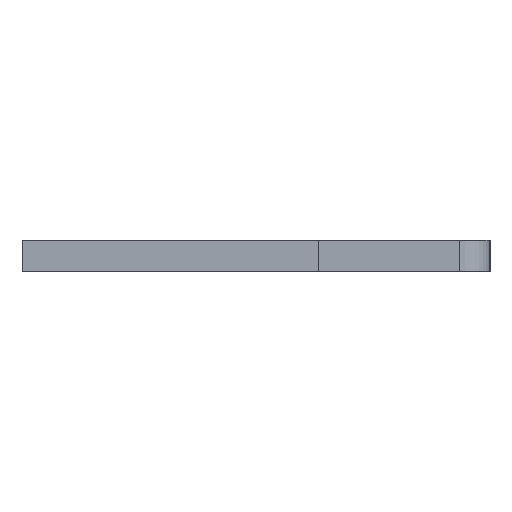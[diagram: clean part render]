
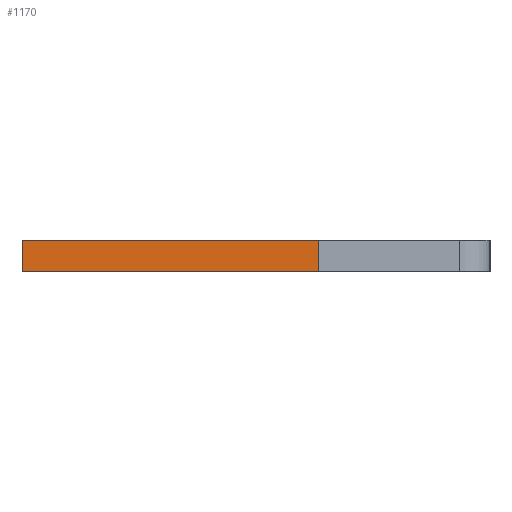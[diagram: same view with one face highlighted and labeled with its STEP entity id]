
A CAD part, left-side view. The second image highlights one B-rep face of the part: STEP entity #1170.
In plain terms, the highlighted face is planar.
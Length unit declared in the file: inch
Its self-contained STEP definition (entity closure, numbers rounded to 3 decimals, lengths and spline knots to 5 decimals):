
#12 = PLANE ( 'NONE',  #381 ) ;
#14 = EDGE_CURVE ( 'NONE', #1095, #1069, #570, .T. ) ;
#95 = DIRECTION ( 'NONE',  ( 0., 1., 0. ) ) ;
#118 = DIRECTION ( 'NONE',  ( 0., 1., 0. ) ) ;
#135 = VECTOR ( 'NONE', #1110, 39.37008 ) ;
#197 = DIRECTION ( 'NONE',  ( 1., 0., 0. ) ) ;
#214 = CARTESIAN_POINT ( 'NONE',  ( 0.01, -0.04, -0.04 ) ) ;
#228 = VECTOR ( 'NONE', #118, 39.37008 ) ;
#239 = DIRECTION ( 'NONE',  ( -1., 0., 0. ) ) ;
#285 = CARTESIAN_POINT ( 'NONE',  ( 0.01, 0.15, -0.04 ) ) ;
#304 = FACE_OUTER_BOUND ( 'NONE', #419, .T. ) ;
#349 = ORIENTED_EDGE ( 'NONE', *, *, #484, .F. ) ;
#381 = AXIS2_PLACEMENT_3D ( 'NONE', #285, #1115, #197 ) ;
#419 = EDGE_LOOP ( 'NONE', ( #851, #349, #1166, #586 ) ) ;
#484 = EDGE_CURVE ( 'NONE', #1089, #1069, #775, .T. ) ;
#508 = CARTESIAN_POINT ( 'NONE',  ( 0.01, 0.15, -0.04 ) ) ;
#570 = LINE ( 'NONE', #932, #809 ) ;
#586 = ORIENTED_EDGE ( 'NONE', *, *, #738, .T. ) ;
#591 = LINE ( 'NONE', #664, #228 ) ;
#638 = CARTESIAN_POINT ( 'NONE',  ( 0.01, -0.04, -0.04 ) ) ;
#664 = CARTESIAN_POINT ( 'NONE',  ( 0.01, 0.15, -0.04 ) ) ;
#681 = LINE ( 'NONE', #214, #135 ) ;
#738 = EDGE_CURVE ( 'NONE', #755, #1095, #681, .T. ) ;
#755 = VERTEX_POINT ( 'NONE', #638 ) ;
#775 = LINE ( 'NONE', #508, #884 ) ;
#809 = VECTOR ( 'NONE', #95, 39.37008 ) ;
#851 = ORIENTED_EDGE ( 'NONE', *, *, #14, .T. ) ;
#861 = CARTESIAN_POINT ( 'NONE',  ( -0.01, 0.15, -0.04 ) ) ;
#884 = VECTOR ( 'NONE', #239, 39.37008 ) ;
#903 = CARTESIAN_POINT ( 'NONE',  ( 0.01, 0.15, -0.04 ) ) ;
#932 = CARTESIAN_POINT ( 'NONE',  ( -0.01, 0.15, -0.04 ) ) ;
#993 = CARTESIAN_POINT ( 'NONE',  ( -0.01, -0.04, -0.04 ) ) ;
#1069 = VERTEX_POINT ( 'NONE', #861 ) ;
#1089 = VERTEX_POINT ( 'NONE', #903 ) ;
#1095 = VERTEX_POINT ( 'NONE', #993 ) ;
#1110 = DIRECTION ( 'NONE',  ( -1., 0., 0. ) ) ;
#1115 = DIRECTION ( 'NONE',  ( 0., 0., 1. ) ) ;
#1166 = ORIENTED_EDGE ( 'NONE', *, *, #1174, .F. ) ;
#1170 = ADVANCED_FACE ( 'NONE', ( #304 ), #12, .F. ) ;
#1174 = EDGE_CURVE ( 'NONE', #755, #1089, #591, .T. ) ;
